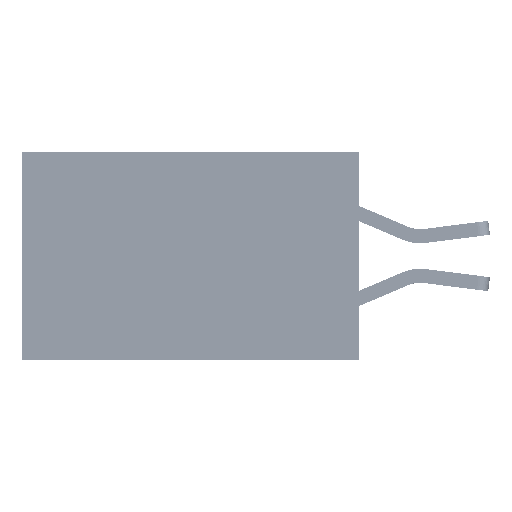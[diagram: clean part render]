
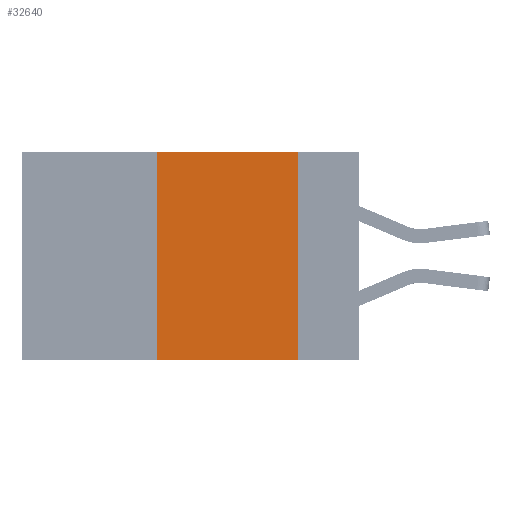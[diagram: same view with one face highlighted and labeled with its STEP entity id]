
A CAD part, left-side view. The second image highlights one B-rep face of the part: STEP entity #32640.
In plain terms, the highlighted planar face has unit normal (-1, 0, 0).
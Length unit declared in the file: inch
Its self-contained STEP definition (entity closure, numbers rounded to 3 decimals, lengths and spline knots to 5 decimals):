
#64 = PLANE ( 'NONE',  #11489 ) ;
#275 = EDGE_CURVE ( 'NONE', #23404, #3125, #12780, .T. ) ;
#1004 = ORIENTED_EDGE ( 'NONE', *, *, #1438, .T. ) ;
#1438 = EDGE_CURVE ( 'NONE', #26186, #3125, #19850, .T. ) ;
#3125 = VERTEX_POINT ( 'NONE', #15049 ) ;
#3480 = DIRECTION ( 'NONE',  ( 0., 0., -1. ) ) ;
#10127 = LINE ( 'NONE', #10232, #26480 ) ;
#10232 = CARTESIAN_POINT ( 'NONE',  ( 0., 0.36, 0. ) ) ;
#10641 = DIRECTION ( 'NONE',  ( 0., -1., 0. ) ) ;
#11489 = AXIS2_PLACEMENT_3D ( 'NONE', #36104, #23200, #3480 ) ;
#12462 = CARTESIAN_POINT ( 'NONE',  ( 0., 0.36, -0.37 ) ) ;
#12780 = LINE ( 'NONE', #34078, #36721 ) ;
#13531 = DIRECTION ( 'NONE',  ( 0., 0., 1. ) ) ;
#15049 = CARTESIAN_POINT ( 'NONE',  ( 0., 0.11, -0.37 ) ) ;
#17061 = CARTESIAN_POINT ( 'NONE',  ( 0., 0.6, 0. ) ) ;
#18307 = EDGE_CURVE ( 'NONE', #31984, #23404, #39148, .T. ) ;
#19724 = DIRECTION ( 'NONE',  ( 0., -1., 0. ) ) ;
#19850 = LINE ( 'NONE', #23012, #27485 ) ;
#20124 = CARTESIAN_POINT ( 'NONE',  ( 0., 0.36, 0. ) ) ;
#20669 = CARTESIAN_POINT ( 'NONE',  ( 0., 0.11, 0. ) ) ;
#23012 = CARTESIAN_POINT ( 'NONE',  ( 0., 0.6, -0.37 ) ) ;
#23200 = DIRECTION ( 'NONE',  ( 1., 0., 0. ) ) ;
#23404 = VERTEX_POINT ( 'NONE', #20669 ) ;
#24262 = ORIENTED_EDGE ( 'NONE', *, *, #18307, .F. ) ;
#26186 = VERTEX_POINT ( 'NONE', #12462 ) ;
#26293 = ORIENTED_EDGE ( 'NONE', *, *, #31947, .F. ) ;
#26480 = VECTOR ( 'NONE', #13531, 39.37008 ) ;
#27485 = VECTOR ( 'NONE', #19724, 39.37008 ) ;
#28621 = EDGE_LOOP ( 'NONE', ( #40515, #24262, #26293, #1004 ) ) ;
#30507 = VECTOR ( 'NONE', #10641, 39.37008 ) ;
#30819 = DIRECTION ( 'NONE',  ( 0., 0., -1. ) ) ;
#31947 = EDGE_CURVE ( 'NONE', #26186, #31984, #10127, .T. ) ;
#31984 = VERTEX_POINT ( 'NONE', #20124 ) ;
#32640 = ADVANCED_FACE ( 'NONE', ( #34527 ), #64, .F. ) ;
#34078 = CARTESIAN_POINT ( 'NONE',  ( 0., 0.11, 0. ) ) ;
#34527 = FACE_OUTER_BOUND ( 'NONE', #28621, .T. ) ;
#36104 = CARTESIAN_POINT ( 'NONE',  ( 0., 0.6, 0. ) ) ;
#36721 = VECTOR ( 'NONE', #30819, 39.37008 ) ;
#39148 = LINE ( 'NONE', #17061, #30507 ) ;
#40515 = ORIENTED_EDGE ( 'NONE', *, *, #275, .F. ) ;
